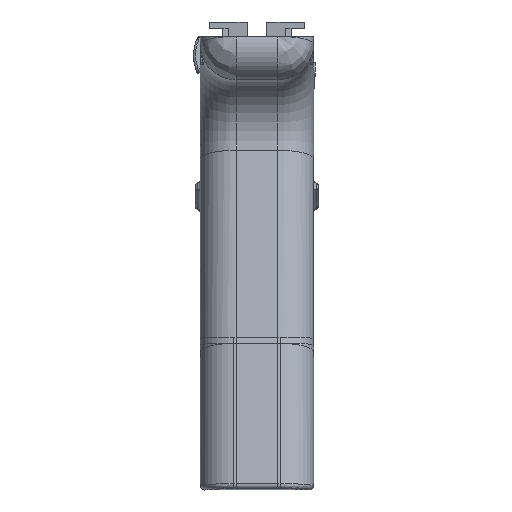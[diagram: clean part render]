
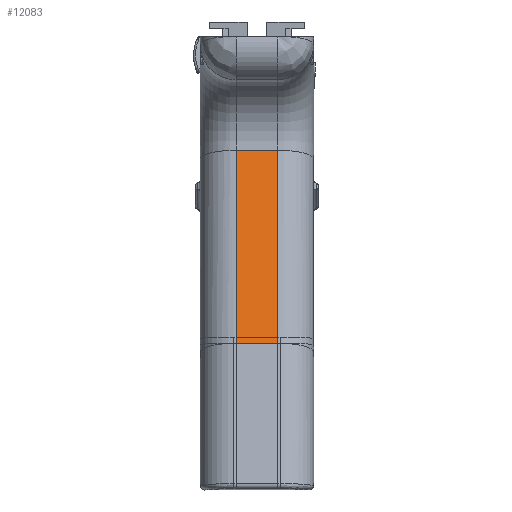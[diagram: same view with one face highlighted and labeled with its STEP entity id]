
A CAD part, front view. The second image highlights one B-rep face of the part: STEP entity #12083.
In plain terms, the highlighted face is planar.
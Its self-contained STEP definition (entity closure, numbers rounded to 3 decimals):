
#928=PLANE('',#13206);
#1506=FACE_OUTER_BOUND('',#2198,.T.);
#2198=EDGE_LOOP('',(#10665,#10666,#10667,#10668));
#3128=LINE('',#21801,#4216);
#3285=LINE('',#22656,#4373);
#3286=LINE('',#22659,#4374);
#3287=LINE('',#22660,#4375);
#4216=VECTOR('',#15725,10.);
#4373=VECTOR('',#16130,10.);
#4374=VECTOR('',#16133,10.);
#4375=VECTOR('',#16134,10.);
#5705=VERTEX_POINT('',#21797);
#5706=VERTEX_POINT('',#21799);
#5847=VERTEX_POINT('',#22634);
#5850=VERTEX_POINT('',#22658);
#7292=EDGE_CURVE('',#5705,#5706,#3128,.T.);
#7519=EDGE_CURVE('',#5705,#5847,#3285,.T.);
#7520=EDGE_CURVE('',#5850,#5706,#3286,.T.);
#7521=EDGE_CURVE('',#5847,#5850,#3287,.T.);
#10665=ORIENTED_EDGE('',*,*,#7520,.F.);
#10666=ORIENTED_EDGE('',*,*,#7521,.F.);
#10667=ORIENTED_EDGE('',*,*,#7519,.F.);
#10668=ORIENTED_EDGE('',*,*,#7292,.T.);
#12083=ADVANCED_FACE('',(#1506),#928,.T.);
#13206=AXIS2_PLACEMENT_3D('',#22657,#16131,#16132);
#15725=DIRECTION('',(0.,-0.249,0.969));
#16130=DIRECTION('',(-1.,0.,0.));
#16131=DIRECTION('center_axis',(0.,-0.969,
-0.249));
#16132=DIRECTION('ref_axis',(0.,-0.249,0.969));
#16133=DIRECTION('',(1.,0.,0.));
#16134=DIRECTION('',(0.,-0.249,0.969));
#21797=CARTESIAN_POINT('',(13.45,-71.634,19.877));
#21799=CARTESIAN_POINT('',(13.45,-83.628,66.536));
#21801=CARTESIAN_POINT('',(13.45,-83.554,66.245));
#22634=CARTESIAN_POINT('',(3.45,-71.634,19.877));
#22656=CARTESIAN_POINT('',(22.175,-71.634,19.877));
#22657=CARTESIAN_POINT('Origin',(22.175,-71.634,19.877));
#22658=CARTESIAN_POINT('',(3.45,-83.628,66.536));
#22659=CARTESIAN_POINT('',(22.175,-83.628,66.536));
#22660=CARTESIAN_POINT('',(3.45,-83.554,66.245));
